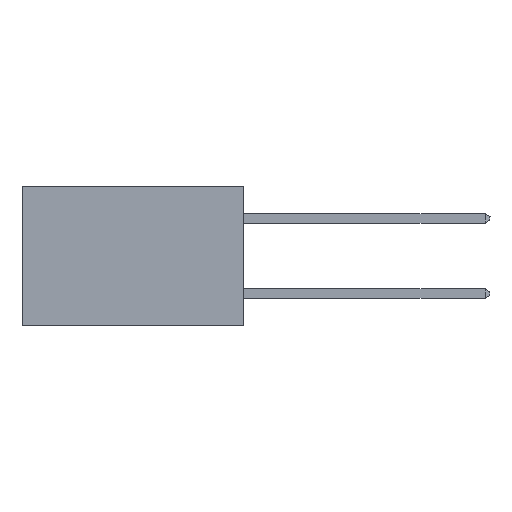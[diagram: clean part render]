
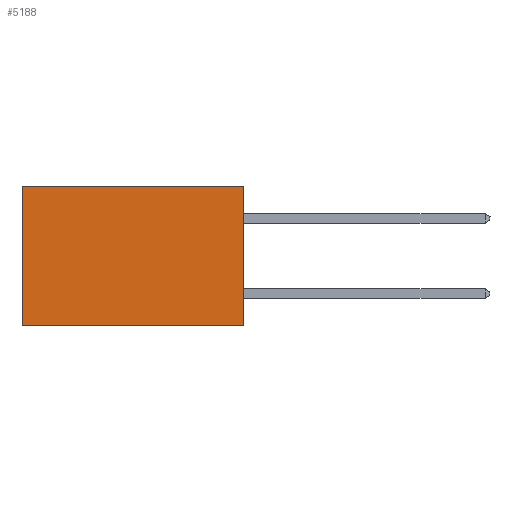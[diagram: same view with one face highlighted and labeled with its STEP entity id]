
A CAD part, left-side view. The second image highlights one B-rep face of the part: STEP entity #5188.
In plain terms, the highlighted planar face has unit normal (-1, 0, 0).
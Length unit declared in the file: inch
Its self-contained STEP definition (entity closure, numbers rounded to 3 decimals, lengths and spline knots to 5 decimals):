
#145 = CARTESIAN_POINT ( 'NONE',  ( 0.277, 0., 0. ) ) ;
#337 = EDGE_CURVE ( 'NONE', #3146, #8948, #4248, .T. ) ;
#399 = VECTOR ( 'NONE', #13188, 39.37008 ) ;
#796 = CARTESIAN_POINT ( 'NONE',  ( 0.277, 0.59, -0.37 ) ) ;
#1086 = CARTESIAN_POINT ( 'NONE',  ( 0.277, 0., -0.37 ) ) ;
#2273 = VECTOR ( 'NONE', #8868, 39.37008 ) ;
#3146 = VERTEX_POINT ( 'NONE', #145 ) ;
#3360 = VERTEX_POINT ( 'NONE', #796 ) ;
#4176 = EDGE_CURVE ( 'NONE', #3146, #6053, #9062, .T. ) ;
#4248 = LINE ( 'NONE', #13088, #10475 ) ;
#4381 = DIRECTION ( 'NONE',  ( 0., 0., -1. ) ) ;
#4458 = DIRECTION ( 'NONE',  ( 0., 0., -1. ) ) ;
#5028 = AXIS2_PLACEMENT_3D ( 'NONE', #8055, #8033, #8018 ) ;
#5188 = ADVANCED_FACE ( 'NONE', ( #14468 ), #8154, .F. ) ;
#6053 = VERTEX_POINT ( 'NONE', #10228 ) ;
#8018 = DIRECTION ( 'NONE',  ( 0., 0., -1. ) ) ;
#8033 = DIRECTION ( 'NONE',  ( 1., 0., 0. ) ) ;
#8055 = CARTESIAN_POINT ( 'NONE',  ( 0.277, 0., -0.37 ) ) ;
#8154 = PLANE ( 'NONE',  #5028 ) ;
#8287 = ORIENTED_EDGE ( 'NONE', *, *, #4176, .T. ) ;
#8530 = ORIENTED_EDGE ( 'NONE', *, *, #337, .F. ) ;
#8597 = VECTOR ( 'NONE', #4458, 39.37008 ) ;
#8868 = DIRECTION ( 'NONE',  ( 0., 1., 0. ) ) ;
#8948 = VERTEX_POINT ( 'NONE', #1086 ) ;
#9028 = ORIENTED_EDGE ( 'NONE', *, *, #15206, .F. ) ;
#9062 = LINE ( 'NONE', #9729, #2273 ) ;
#9729 = CARTESIAN_POINT ( 'NONE',  ( 0.277, 0., 0. ) ) ;
#9994 = EDGE_CURVE ( 'NONE', #6053, #3360, #11841, .T. ) ;
#10228 = CARTESIAN_POINT ( 'NONE',  ( 0.277, 0.59, 0. ) ) ;
#10427 = LINE ( 'NONE', #11998, #399 ) ;
#10475 = VECTOR ( 'NONE', #4381, 39.37008 ) ;
#10579 = ORIENTED_EDGE ( 'NONE', *, *, #9994, .T. ) ;
#11841 = LINE ( 'NONE', #13116, #8597 ) ;
#11998 = CARTESIAN_POINT ( 'NONE',  ( 0.277, 0., -0.37 ) ) ;
#12113 = EDGE_LOOP ( 'NONE', ( #10579, #9028, #8530, #8287 ) ) ;
#13088 = CARTESIAN_POINT ( 'NONE',  ( 0.277, 0., -0.37 ) ) ;
#13116 = CARTESIAN_POINT ( 'NONE',  ( 0.277, 0.59, -0.37 ) ) ;
#13188 = DIRECTION ( 'NONE',  ( 0., 1., 0. ) ) ;
#14468 = FACE_OUTER_BOUND ( 'NONE', #12113, .T. ) ;
#15206 = EDGE_CURVE ( 'NONE', #8948, #3360, #10427, .T. ) ;
